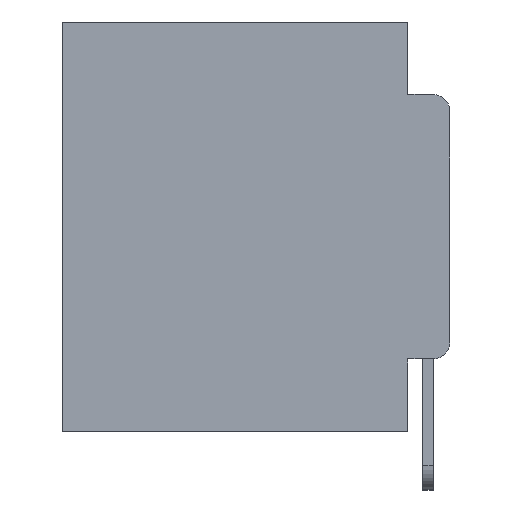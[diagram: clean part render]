
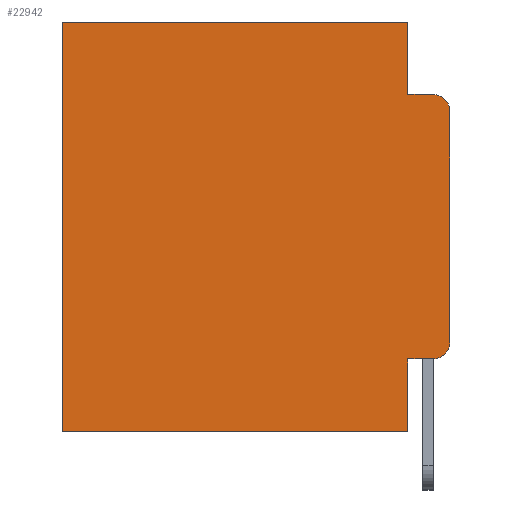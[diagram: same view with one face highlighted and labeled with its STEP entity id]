
A CAD part, left-side view. The second image highlights one B-rep face of the part: STEP entity #22942.
In plain terms, the highlighted planar face has unit normal (-1, 0, 0).
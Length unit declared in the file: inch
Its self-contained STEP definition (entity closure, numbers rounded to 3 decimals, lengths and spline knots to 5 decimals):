
#279 = VECTOR ( 'NONE', #28047, 39.37008 ) ;
#1233 = CARTESIAN_POINT ( 'NONE',  ( 0.298, 0.02, -0.3915 ) ) ;
#1678 = ORIENTED_EDGE ( 'NONE', *, *, #13698, .F. ) ;
#2101 = ORIENTED_EDGE ( 'NONE', *, *, #14898, .F. ) ;
#2240 = VECTOR ( 'NONE', #17323, 39.37008 ) ;
#2628 = AXIS2_PLACEMENT_3D ( 'NONE', #1233, #23668, #27800 ) ;
#3417 = DIRECTION ( 'NONE',  ( 0., 1., 0. ) ) ;
#3988 = VERTEX_POINT ( 'NONE', #16961 ) ;
#4108 = VECTOR ( 'NONE', #3417, 39.37008 ) ;
#5051 = DIRECTION ( 'NONE',  ( 0., 1., 0. ) ) ;
#5613 = CARTESIAN_POINT ( 'NONE',  ( 0.298, 0.051, 0. ) ) ;
#5980 = FACE_OUTER_BOUND ( 'NONE', #23677, .T. ) ;
#6086 = CARTESIAN_POINT ( 'NONE',  ( 0.298, 0.051, -0.4115 ) ) ;
#6444 = CARTESIAN_POINT ( 'NONE',  ( 0.298, 0.051, 0. ) ) ;
#6552 = VERTEX_POINT ( 'NONE', #24056 ) ;
#6925 = DIRECTION ( 'NONE',  ( 0., 0., -1. ) ) ;
#7381 = EDGE_CURVE ( 'NONE', #7477, #27782, #25459, .T. ) ;
#7388 = CARTESIAN_POINT ( 'NONE',  ( 0.298, 0.051, -0.0885 ) ) ;
#7477 = VERTEX_POINT ( 'NONE', #26204 ) ;
#7498 = VERTEX_POINT ( 'NONE', #24093 ) ;
#7506 = DIRECTION ( 'NONE',  ( 0., 0., -1. ) ) ;
#7542 = CARTESIAN_POINT ( 'NONE',  ( 0.298, 0.051, -0.0885 ) ) ;
#8702 = VECTOR ( 'NONE', #28279, 39.37008 ) ;
#8852 = ORIENTED_EDGE ( 'NONE', *, *, #12211, .T. ) ;
#8984 = VERTEX_POINT ( 'NONE', #10621 ) ;
#9282 = CARTESIAN_POINT ( 'NONE',  ( 0.298, 0., 0. ) ) ;
#9387 = EDGE_CURVE ( 'NONE', #19765, #25336, #25527, .T. ) ;
#9692 = EDGE_CURVE ( 'NONE', #11604, #27782, #11383, .T. ) ;
#9767 = VECTOR ( 'NONE', #27154, 39.37008 ) ;
#9883 = ORIENTED_EDGE ( 'NONE', *, *, #14552, .F. ) ;
#10621 = CARTESIAN_POINT ( 'NONE',  ( 0.298, 0., -0.3915 ) ) ;
#11170 = CARTESIAN_POINT ( 'NONE',  ( 0.298, 0., 0. ) ) ;
#11383 = LINE ( 'NONE', #7542, #15854 ) ;
#11471 = VECTOR ( 'NONE', #5051, 39.37008 ) ;
#11518 = VECTOR ( 'NONE', #7506, 39.37008 ) ;
#11604 = VERTEX_POINT ( 'NONE', #7388 ) ;
#12211 = EDGE_CURVE ( 'NONE', #25424, #3988, #23667, .T. ) ;
#12576 = DIRECTION ( 'NONE',  ( -1., 0., 0. ) ) ;
#12637 = CARTESIAN_POINT ( 'NONE',  ( 0.298, 0.051, -0.4115 ) ) ;
#13698 = EDGE_CURVE ( 'NONE', #7477, #8984, #24629, .T. ) ;
#14230 = ORIENTED_EDGE ( 'NONE', *, *, #7381, .T. ) ;
#14552 = EDGE_CURVE ( 'NONE', #6552, #11604, #18662, .T. ) ;
#14745 = CARTESIAN_POINT ( 'NONE',  ( 0.298, 0.02, -0.4115 ) ) ;
#14804 = LINE ( 'NONE', #21127, #4108 ) ;
#14898 = EDGE_CURVE ( 'NONE', #19765, #7498, #26955, .T. ) ;
#15199 = ORIENTED_EDGE ( 'NONE', *, *, #28526, .T. ) ;
#15854 = VECTOR ( 'NONE', #26857, 39.37008 ) ;
#15937 = LINE ( 'NONE', #9282, #11471 ) ;
#16961 = CARTESIAN_POINT ( 'NONE',  ( 0.298, 0.473, -0.5 ) ) ;
#17224 = CARTESIAN_POINT ( 'NONE',  ( 0.298, 0.473, 0. ) ) ;
#17323 = DIRECTION ( 'NONE',  ( 0., 0., -1. ) ) ;
#17617 = ORIENTED_EDGE ( 'NONE', *, *, #9692, .F. ) ;
#18270 = CIRCLE ( 'NONE', #2628, 0.02 ) ;
#18378 = AXIS2_PLACEMENT_3D ( 'NONE', #25679, #12576, #18981 ) ;
#18662 = LINE ( 'NONE', #5613, #9767 ) ;
#18981 = DIRECTION ( 'NONE',  ( 0., 0., -1. ) ) ;
#19765 = VERTEX_POINT ( 'NONE', #6086 ) ;
#19838 = ORIENTED_EDGE ( 'NONE', *, *, #25829, .F. ) ;
#20825 = ORIENTED_EDGE ( 'NONE', *, *, #24204, .T. ) ;
#21127 = CARTESIAN_POINT ( 'NONE',  ( 0.298, 0., -0.5 ) ) ;
#22227 = PLANE ( 'NONE',  #28132 ) ;
#22942 = ADVANCED_FACE ( 'NONE', ( #5980 ), #22227, .F. ) ;
#22997 = CARTESIAN_POINT ( 'NONE',  ( 0.298, 0., 0. ) ) ;
#23667 = LINE ( 'NONE', #17224, #2240 ) ;
#23668 = DIRECTION ( 'NONE',  ( -1., 0., 0. ) ) ;
#23677 = EDGE_LOOP ( 'NONE', ( #1678, #14230, #17617, #9883, #15199, #8852, #19838, #2101, #26382, #20825 ) ) ;
#24056 = CARTESIAN_POINT ( 'NONE',  ( 0.298, 0.051, 0. ) ) ;
#24093 = CARTESIAN_POINT ( 'NONE',  ( 0.298, 0.051, -0.5 ) ) ;
#24204 = EDGE_CURVE ( 'NONE', #25336, #8984, #18270, .T. ) ;
#24629 = LINE ( 'NONE', #22997, #11518 ) ;
#25336 = VERTEX_POINT ( 'NONE', #14745 ) ;
#25424 = VERTEX_POINT ( 'NONE', #28220 ) ;
#25459 = CIRCLE ( 'NONE', #18378, 0.02 ) ;
#25527 = LINE ( 'NONE', #12637, #279 ) ;
#25679 = CARTESIAN_POINT ( 'NONE',  ( 0.298, 0.02, -0.1085 ) ) ;
#25829 = EDGE_CURVE ( 'NONE', #7498, #3988, #14804, .T. ) ;
#26204 = CARTESIAN_POINT ( 'NONE',  ( 0.298, 0., -0.1085 ) ) ;
#26382 = ORIENTED_EDGE ( 'NONE', *, *, #9387, .T. ) ;
#26771 = DIRECTION ( 'NONE',  ( 1., 0., 0. ) ) ;
#26857 = DIRECTION ( 'NONE',  ( 0., -1., 0. ) ) ;
#26955 = LINE ( 'NONE', #6444, #8702 ) ;
#27140 = CARTESIAN_POINT ( 'NONE',  ( 0.298, 0.02, -0.0885 ) ) ;
#27154 = DIRECTION ( 'NONE',  ( 0., 0., -1. ) ) ;
#27782 = VERTEX_POINT ( 'NONE', #27140 ) ;
#27800 = DIRECTION ( 'NONE',  ( 0., 0., -1. ) ) ;
#28047 = DIRECTION ( 'NONE',  ( 0., -1., 0. ) ) ;
#28132 = AXIS2_PLACEMENT_3D ( 'NONE', #11170, #26771, #6925 ) ;
#28220 = CARTESIAN_POINT ( 'NONE',  ( 0.298, 0.473, 0. ) ) ;
#28279 = DIRECTION ( 'NONE',  ( 0., 0., -1. ) ) ;
#28526 = EDGE_CURVE ( 'NONE', #6552, #25424, #15937, .T. ) ;
